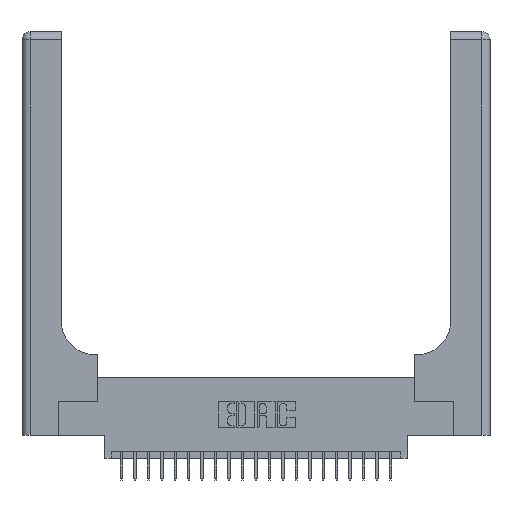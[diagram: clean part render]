
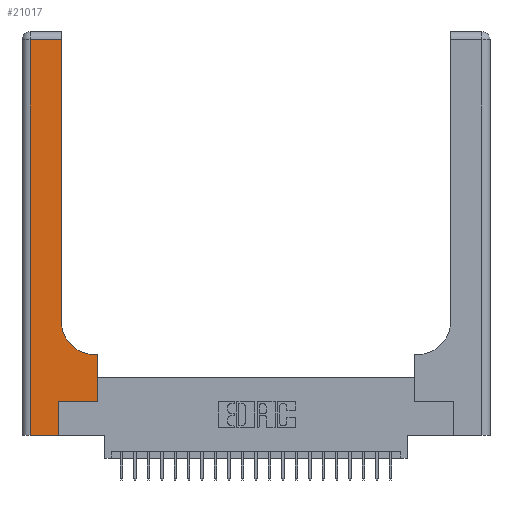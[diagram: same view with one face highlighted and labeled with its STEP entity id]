
A CAD part, top view. The second image highlights one B-rep face of the part: STEP entity #21017.
In plain terms, the highlighted planar face has unit normal (0, 0, 1).
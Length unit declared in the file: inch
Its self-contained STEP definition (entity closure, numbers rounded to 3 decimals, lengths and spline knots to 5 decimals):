
#378 = ORIENTED_EDGE ( 'NONE', *, *, #15893, .T. ) ;
#520 = DIRECTION ( 'NONE',  ( 0., 0., -1. ) ) ;
#858 = DIRECTION ( 'NONE',  ( 0., 1., 0. ) ) ;
#1190 = CARTESIAN_POINT ( 'NONE',  ( 0.269, 0., 0.37 ) ) ;
#1250 = VECTOR ( 'NONE', #10015, 39.37008 ) ;
#1711 = VERTEX_POINT ( 'NONE', #5474 ) ;
#2051 = EDGE_LOOP ( 'NONE', ( #5601, #14395, #12879, #11352, #18655, #378, #6957, #7159, #16713 ) ) ;
#2361 = VECTOR ( 'NONE', #6471, 39.37008 ) ;
#3521 = VERTEX_POINT ( 'NONE', #16127 ) ;
#5295 = CARTESIAN_POINT ( 'NONE',  ( 0.5415, 0.6, 0.37 ) ) ;
#5474 = CARTESIAN_POINT ( 'NONE',  ( 0.269, 0.25, 0.37 ) ) ;
#5601 = ORIENTED_EDGE ( 'NONE', *, *, #7929, .T. ) ;
#5671 = CARTESIAN_POINT ( 'NONE',  ( 0.269, 0., 0.37 ) ) ;
#5764 = LINE ( 'NONE', #12508, #15374 ) ;
#6024 = CARTESIAN_POINT ( 'NONE',  ( 0.2915, 0.85, 0.37 ) ) ;
#6097 = FACE_OUTER_BOUND ( 'NONE', #2051, .T. ) ;
#6128 = CARTESIAN_POINT ( 'NONE',  ( 0.06, 3., 0.37 ) ) ;
#6203 = CARTESIAN_POINT ( 'NONE',  ( 0.5585, 0.25, 0.37 ) ) ;
#6471 = DIRECTION ( 'NONE',  ( 1., 0., 0. ) ) ;
#6480 = AXIS2_PLACEMENT_3D ( 'NONE', #9033, #22240, #10961 ) ;
#6516 = VERTEX_POINT ( 'NONE', #17431 ) ;
#6702 = DIRECTION ( 'NONE',  ( -1., 0., 0. ) ) ;
#6782 = EDGE_CURVE ( 'NONE', #6516, #17534, #12360, .T. ) ;
#6957 = ORIENTED_EDGE ( 'NONE', *, *, #14410, .T. ) ;
#7159 = ORIENTED_EDGE ( 'NONE', *, *, #14550, .T. ) ;
#7253 = VECTOR ( 'NONE', #24152, 39.37008 ) ;
#7726 = VERTEX_POINT ( 'NONE', #6024 ) ;
#7929 = EDGE_CURVE ( 'NONE', #7726, #3521, #20458, .T. ) ;
#8219 = PLANE ( 'NONE',  #15131 ) ;
#9033 = CARTESIAN_POINT ( 'NONE',  ( 0.5415, 0.85, 0.37 ) ) ;
#9804 = VECTOR ( 'NONE', #858, 39.37008 ) ;
#10015 = DIRECTION ( 'NONE',  ( 0., -1., 0. ) ) ;
#10092 = CARTESIAN_POINT ( 'NONE',  ( 0.5585, 0.25, 0.37 ) ) ;
#10237 = LINE ( 'NONE', #1190, #14717 ) ;
#10285 = CARTESIAN_POINT ( 'NONE',  ( 0., 2.94, 0.37 ) ) ;
#10379 = VERTEX_POINT ( 'NONE', #5295 ) ;
#10961 = DIRECTION ( 'NONE',  ( 1., 0., 0. ) ) ;
#10962 = CARTESIAN_POINT ( 'NONE',  ( 0., 0., 0.37 ) ) ;
#11352 = ORIENTED_EDGE ( 'NONE', *, *, #6782, .T. ) ;
#12212 = DIRECTION ( 'NONE',  ( -1., 0., 0. ) ) ;
#12288 = CARTESIAN_POINT ( 'NONE',  ( 0.269, 0.25, 0.37 ) ) ;
#12298 = CARTESIAN_POINT ( 'NONE',  ( 0.5585, 0.6, 0.37 ) ) ;
#12360 = LINE ( 'NONE', #10962, #7253 ) ;
#12508 = CARTESIAN_POINT ( 'NONE',  ( 0.2915, 0.6, 0.37 ) ) ;
#12832 = DIRECTION ( 'NONE',  ( 0., 1., 0. ) ) ;
#12879 = ORIENTED_EDGE ( 'NONE', *, *, #20571, .T. ) ;
#13019 = LINE ( 'NONE', #10285, #16860 ) ;
#13935 = DIRECTION ( 'NONE',  ( 0., 1., 0. ) ) ;
#13997 = DIRECTION ( 'NONE',  ( -1., 0., 0. ) ) ;
#14395 = ORIENTED_EDGE ( 'NONE', *, *, #20040, .T. ) ;
#14410 = EDGE_CURVE ( 'NONE', #16410, #19509, #23280, .T. ) ;
#14475 = VECTOR ( 'NONE', #13935, 39.37008 ) ;
#14550 = EDGE_CURVE ( 'NONE', #19509, #10379, #5764, .T. ) ;
#14717 = VECTOR ( 'NONE', #12832, 39.37008 ) ;
#15130 = CARTESIAN_POINT ( 'NONE',  ( 0.06, 2.94, 0.37 ) ) ;
#15131 = AXIS2_PLACEMENT_3D ( 'NONE', #17700, #520, #13997 ) ;
#15374 = VECTOR ( 'NONE', #6702, 39.37008 ) ;
#15893 = EDGE_CURVE ( 'NONE', #1711, #16410, #18233, .T. ) ;
#16127 = CARTESIAN_POINT ( 'NONE',  ( 0.2915, 2.94, 0.37 ) ) ;
#16410 = VERTEX_POINT ( 'NONE', #6203 ) ;
#16713 = ORIENTED_EDGE ( 'NONE', *, *, #24052, .T. ) ;
#16860 = VECTOR ( 'NONE', #12212, 39.37008 ) ;
#17169 = LINE ( 'NONE', #6128, #1250 ) ;
#17431 = CARTESIAN_POINT ( 'NONE',  ( 0.06, 0., 0.37 ) ) ;
#17534 = VERTEX_POINT ( 'NONE', #5671 ) ;
#17700 = CARTESIAN_POINT ( 'NONE',  ( 0., 3., 0.37 ) ) ;
#18155 = VERTEX_POINT ( 'NONE', #15130 ) ;
#18233 = LINE ( 'NONE', #12288, #2361 ) ;
#18655 = ORIENTED_EDGE ( 'NONE', *, *, #23454, .T. ) ;
#19509 = VERTEX_POINT ( 'NONE', #12298 ) ;
#20040 = EDGE_CURVE ( 'NONE', #3521, #18155, #13019, .T. ) ;
#20458 = LINE ( 'NONE', #23677, #9804 ) ;
#20571 = EDGE_CURVE ( 'NONE', #18155, #6516, #17169, .T. ) ;
#21017 = ADVANCED_FACE ( 'NONE', ( #6097 ), #8219, .F. ) ;
#22240 = DIRECTION ( 'NONE',  ( 0., 0., -1. ) ) ;
#22310 = CIRCLE ( 'NONE', #6480, 0.25 ) ;
#23280 = LINE ( 'NONE', #10092, #14475 ) ;
#23454 = EDGE_CURVE ( 'NONE', #17534, #1711, #10237, .T. ) ;
#23677 = CARTESIAN_POINT ( 'NONE',  ( 0.2915, 3., 0.37 ) ) ;
#24052 = EDGE_CURVE ( 'NONE', #10379, #7726, #22310, .T. ) ;
#24152 = DIRECTION ( 'NONE',  ( 1., 0., 0. ) ) ;
